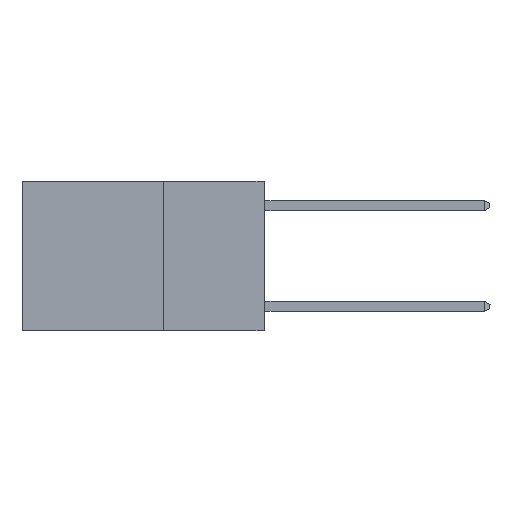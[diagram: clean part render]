
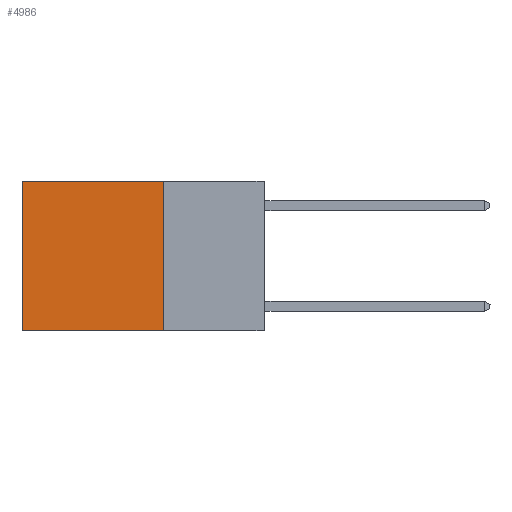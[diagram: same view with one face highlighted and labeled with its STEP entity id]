
A CAD part, left-side view. The second image highlights one B-rep face of the part: STEP entity #4986.
In plain terms, the highlighted planar face has unit normal (-1, 0, 0).
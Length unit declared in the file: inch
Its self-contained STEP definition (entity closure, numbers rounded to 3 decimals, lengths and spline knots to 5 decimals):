
#618 = DIRECTION ( 'NONE',  ( 0., 0., -1. ) ) ;
#2085 = EDGE_CURVE ( 'NONE', #12252, #2101, #7703, .T. ) ;
#2101 = VERTEX_POINT ( 'NONE', #13773 ) ;
#4817 = CARTESIAN_POINT ( 'NONE',  ( 0.2625, 0.25, 0. ) ) ;
#4986 = ADVANCED_FACE ( 'NONE', ( #9105 ), #8008, .F. ) ;
#5715 = DIRECTION ( 'NONE',  ( 0., 0., -1. ) ) ;
#6244 = DIRECTION ( 'NONE',  ( 0., 0., -1. ) ) ;
#7062 = CARTESIAN_POINT ( 'NONE',  ( 0.2625, 0.25, -0.37 ) ) ;
#7426 = LINE ( 'NONE', #4817, #10750 ) ;
#7703 = LINE ( 'NONE', #8081, #15222 ) ;
#8008 = PLANE ( 'NONE',  #13894 ) ;
#8081 = CARTESIAN_POINT ( 'NONE',  ( 0.2625, 0.25, -0.37 ) ) ;
#8326 = VERTEX_POINT ( 'NONE', #18216 ) ;
#8738 = VECTOR ( 'NONE', #13355, 39.37008 ) ;
#9105 = FACE_OUTER_BOUND ( 'NONE', #12094, .T. ) ;
#9454 = DIRECTION ( 'NONE',  ( 1., 0., 0. ) ) ;
#10750 = VECTOR ( 'NONE', #6244, 39.37008 ) ;
#11756 = LINE ( 'NONE', #15566, #15920 ) ;
#11969 = ORIENTED_EDGE ( 'NONE', *, *, #12278, .T. ) ;
#12094 = EDGE_LOOP ( 'NONE', ( #11969, #15690, #12835, #16568 ) ) ;
#12252 = VERTEX_POINT ( 'NONE', #7062 ) ;
#12278 = EDGE_CURVE ( 'NONE', #8326, #2101, #11756, .T. ) ;
#12313 = DIRECTION ( 'NONE',  ( 0., 1., 0. ) ) ;
#12517 = LINE ( 'NONE', #16753, #8738 ) ;
#12835 = ORIENTED_EDGE ( 'NONE', *, *, #16461, .F. ) ;
#13172 = VERTEX_POINT ( 'NONE', #17942 ) ;
#13355 = DIRECTION ( 'NONE',  ( 0., 1., 0. ) ) ;
#13636 = CARTESIAN_POINT ( 'NONE',  ( 0.2625, 0.25, 0. ) ) ;
#13773 = CARTESIAN_POINT ( 'NONE',  ( 0.2625, 0.6, -0.37 ) ) ;
#13894 = AXIS2_PLACEMENT_3D ( 'NONE', #13636, #9454, #618 ) ;
#15222 = VECTOR ( 'NONE', #12313, 39.37008 ) ;
#15566 = CARTESIAN_POINT ( 'NONE',  ( 0.2625, 0.6, 0. ) ) ;
#15690 = ORIENTED_EDGE ( 'NONE', *, *, #2085, .F. ) ;
#15920 = VECTOR ( 'NONE', #5715, 39.37008 ) ;
#16461 = EDGE_CURVE ( 'NONE', #13172, #12252, #7426, .T. ) ;
#16568 = ORIENTED_EDGE ( 'NONE', *, *, #16911, .T. ) ;
#16753 = CARTESIAN_POINT ( 'NONE',  ( 0.2625, 0.25, 0. ) ) ;
#16911 = EDGE_CURVE ( 'NONE', #13172, #8326, #12517, .T. ) ;
#17942 = CARTESIAN_POINT ( 'NONE',  ( 0.2625, 0.25, 0. ) ) ;
#18216 = CARTESIAN_POINT ( 'NONE',  ( 0.2625, 0.6, 0. ) ) ;
